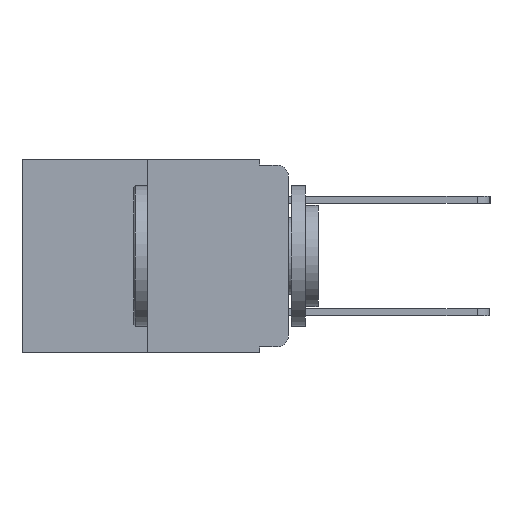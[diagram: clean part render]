
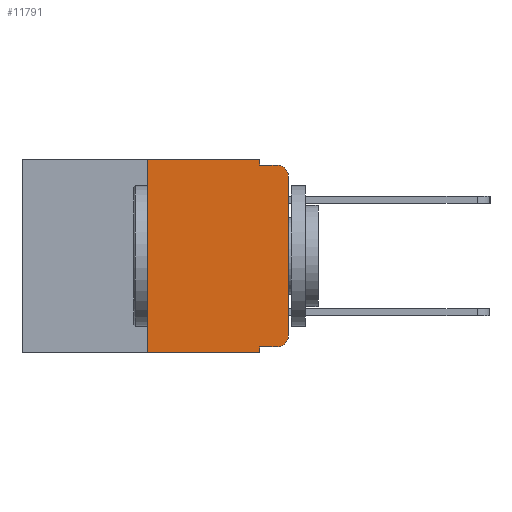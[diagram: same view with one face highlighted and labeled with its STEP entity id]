
A CAD part, left-side view. The second image highlights one B-rep face of the part: STEP entity #11791.
In plain terms, the highlighted planar face has unit normal (-1, 0, 0).
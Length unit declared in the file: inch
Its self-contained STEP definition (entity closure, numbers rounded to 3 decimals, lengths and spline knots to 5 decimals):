
#11 = LINE ( 'NONE', #7295, #7432 ) ;
#200 = PLANE ( 'NONE',  #6348 ) ;
#231 = ORIENTED_EDGE ( 'NONE', *, *, #10215, .T. ) ;
#336 = CARTESIAN_POINT ( 'NONE',  ( 0., 0.25, -0.343 ) ) ;
#479 = EDGE_CURVE ( 'NONE', #4143, #4433, #638, .T. ) ;
#498 = VECTOR ( 'NONE', #3582, 39.37008 ) ;
#553 = ORIENTED_EDGE ( 'NONE', *, *, #9613, .T. ) ;
#614 = VERTEX_POINT ( 'NONE', #7753 ) ;
#638 = LINE ( 'NONE', #2062, #10085 ) ;
#791 = CARTESIAN_POINT ( 'NONE',  ( 0., 0.02, -0.313 ) ) ;
#966 = DIRECTION ( 'NONE',  ( 0., -1., 0. ) ) ;
#1256 = VERTEX_POINT ( 'NONE', #10375 ) ;
#1493 = DIRECTION ( 'NONE',  ( 0., 0., -1. ) ) ;
#1508 = CARTESIAN_POINT ( 'NONE',  ( 0., 0.051, 0. ) ) ;
#1843 = DIRECTION ( 'NONE',  ( 0., 0., -1. ) ) ;
#1876 = EDGE_CURVE ( 'NONE', #6087, #4907, #12144, .T. ) ;
#1987 = CARTESIAN_POINT ( 'NONE',  ( 0., 0., -0.313 ) ) ;
#2002 = CARTESIAN_POINT ( 'NONE',  ( 0., 0.25, 0. ) ) ;
#2033 = DIRECTION ( 'NONE',  ( 0., 0., 1. ) ) ;
#2062 = CARTESIAN_POINT ( 'NONE',  ( 0., 0.25, 0. ) ) ;
#2336 = EDGE_LOOP ( 'NONE', ( #12108, #6010, #6604, #4999, #9866, #3402, #3684, #9177, #231, #553 ) ) ;
#2548 = EDGE_CURVE ( 'NONE', #4907, #9271, #11996, .T. ) ;
#2613 = CARTESIAN_POINT ( 'NONE',  ( 0., 0.473, 0. ) ) ;
#2745 = DIRECTION ( 'NONE',  ( 0., -1., 0. ) ) ;
#3081 = CARTESIAN_POINT ( 'NONE',  ( 0., 0.051, -0.343 ) ) ;
#3204 = EDGE_CURVE ( 'NONE', #1256, #9271, #9746, .T. ) ;
#3263 = CARTESIAN_POINT ( 'NONE',  ( 0., 0.473, 0. ) ) ;
#3278 = VECTOR ( 'NONE', #1493, 39.37008 ) ;
#3321 = CARTESIAN_POINT ( 'NONE',  ( 0., 0.02, -0.01 ) ) ;
#3402 = ORIENTED_EDGE ( 'NONE', *, *, #479, .F. ) ;
#3540 = CARTESIAN_POINT ( 'NONE',  ( 0., 0.051, -0.01 ) ) ;
#3582 = DIRECTION ( 'NONE',  ( 0., -1., 0. ) ) ;
#3684 = ORIENTED_EDGE ( 'NONE', *, *, #9770, .T. ) ;
#3819 = VECTOR ( 'NONE', #5827, 39.37008 ) ;
#3845 = EDGE_CURVE ( 'NONE', #6493, #1256, #6455, .T. ) ;
#4026 = DIRECTION ( 'NONE',  ( -1., 0., 0. ) ) ;
#4143 = VERTEX_POINT ( 'NONE', #336 ) ;
#4227 = DIRECTION ( 'NONE',  ( 0., 0., -1. ) ) ;
#4433 = VERTEX_POINT ( 'NONE', #2002 ) ;
#4546 = DIRECTION ( 'NONE',  ( 0., 0., -1. ) ) ;
#4786 = CARTESIAN_POINT ( 'NONE',  ( 0., 0., 0. ) ) ;
#4907 = VERTEX_POINT ( 'NONE', #3540 ) ;
#4999 = ORIENTED_EDGE ( 'NONE', *, *, #1876, .F. ) ;
#5023 = VECTOR ( 'NONE', #966, 39.37008 ) ;
#5807 = VERTEX_POINT ( 'NONE', #3081 ) ;
#5827 = DIRECTION ( 'NONE',  ( 0., -1., 0. ) ) ;
#6010 = ORIENTED_EDGE ( 'NONE', *, *, #3204, .T. ) ;
#6087 = VERTEX_POINT ( 'NONE', #7160 ) ;
#6285 = VERTEX_POINT ( 'NONE', #9231 ) ;
#6288 = LINE ( 'NONE', #8654, #3819 ) ;
#6348 = AXIS2_PLACEMENT_3D ( 'NONE', #3263, #9712, #4227 ) ;
#6455 = LINE ( 'NONE', #4786, #10981 ) ;
#6493 = VERTEX_POINT ( 'NONE', #1987 ) ;
#6604 = ORIENTED_EDGE ( 'NONE', *, *, #2548, .F. ) ;
#6688 = AXIS2_PLACEMENT_3D ( 'NONE', #9525, #4026, #10429 ) ;
#6730 = FACE_OUTER_BOUND ( 'NONE', #2336, .T. ) ;
#7160 = CARTESIAN_POINT ( 'NONE',  ( 0., 0.051, 0. ) ) ;
#7295 = CARTESIAN_POINT ( 'NONE',  ( 0., 0.051, 0. ) ) ;
#7432 = VECTOR ( 'NONE', #4546, 39.37008 ) ;
#7502 = DIRECTION ( 'NONE',  ( -1., 0., 0. ) ) ;
#7753 = CARTESIAN_POINT ( 'NONE',  ( 0., 0.051, -0.333 ) ) ;
#8318 = CIRCLE ( 'NONE', #10806, 0.02 ) ;
#8440 = VECTOR ( 'NONE', #2745, 39.37008 ) ;
#8654 = CARTESIAN_POINT ( 'NONE',  ( 0., 0.473, -0.343 ) ) ;
#8706 = LINE ( 'NONE', #2613, #498 ) ;
#9177 = ORIENTED_EDGE ( 'NONE', *, *, #12014, .F. ) ;
#9231 = CARTESIAN_POINT ( 'NONE',  ( 0., 0.02, -0.333 ) ) ;
#9271 = VERTEX_POINT ( 'NONE', #3321 ) ;
#9525 = CARTESIAN_POINT ( 'NONE',  ( 0., 0.02, -0.03 ) ) ;
#9613 = EDGE_CURVE ( 'NONE', #6285, #6493, #8318, .T. ) ;
#9712 = DIRECTION ( 'NONE',  ( 1., 0., 0. ) ) ;
#9746 = CIRCLE ( 'NONE', #6688, 0.02 ) ;
#9770 = EDGE_CURVE ( 'NONE', #4143, #5807, #6288, .T. ) ;
#9866 = ORIENTED_EDGE ( 'NONE', *, *, #10754, .F. ) ;
#10085 = VECTOR ( 'NONE', #2033, 39.37008 ) ;
#10215 = EDGE_CURVE ( 'NONE', #614, #6285, #10815, .T. ) ;
#10375 = CARTESIAN_POINT ( 'NONE',  ( 0., 0., -0.03 ) ) ;
#10429 = DIRECTION ( 'NONE',  ( 0., 0., -1. ) ) ;
#10754 = EDGE_CURVE ( 'NONE', #4433, #6087, #8706, .T. ) ;
#10806 = AXIS2_PLACEMENT_3D ( 'NONE', #791, #7502, #1843 ) ;
#10815 = LINE ( 'NONE', #11814, #8440 ) ;
#10981 = VECTOR ( 'NONE', #12100, 39.37008 ) ;
#11791 = ADVANCED_FACE ( 'NONE', ( #6730 ), #200, .F. ) ;
#11814 = CARTESIAN_POINT ( 'NONE',  ( 0., 0.051, -0.333 ) ) ;
#11996 = LINE ( 'NONE', #12131, #5023 ) ;
#12014 = EDGE_CURVE ( 'NONE', #614, #5807, #11, .T. ) ;
#12100 = DIRECTION ( 'NONE',  ( 0., 0., 1. ) ) ;
#12108 = ORIENTED_EDGE ( 'NONE', *, *, #3845, .T. ) ;
#12131 = CARTESIAN_POINT ( 'NONE',  ( 0., 0.051, -0.01 ) ) ;
#12144 = LINE ( 'NONE', #1508, #3278 ) ;
